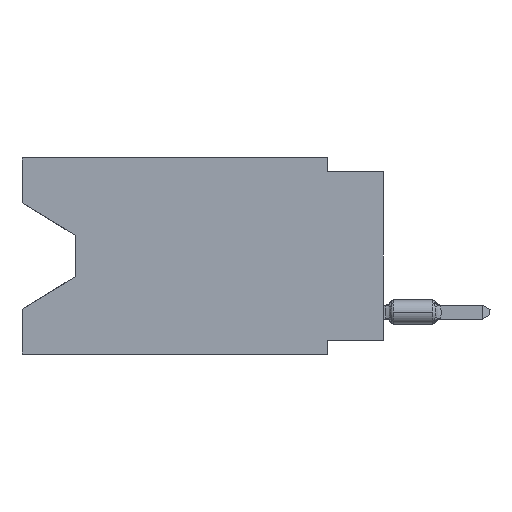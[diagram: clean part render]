
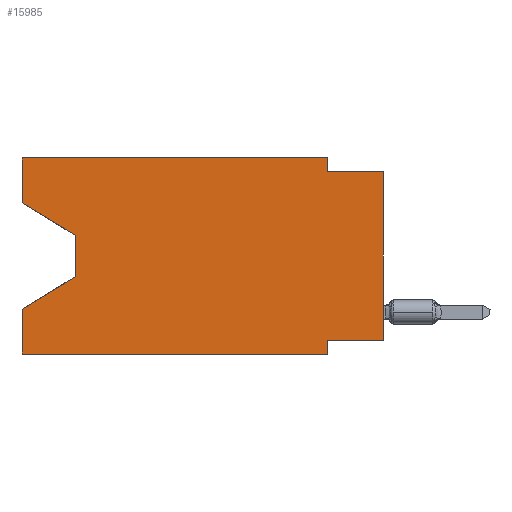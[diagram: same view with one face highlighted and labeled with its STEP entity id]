
A CAD part, left-side view. The second image highlights one B-rep face of the part: STEP entity #15985.
In plain terms, the highlighted planar face has unit normal (-1, 0, 0).
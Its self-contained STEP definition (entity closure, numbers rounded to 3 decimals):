
#483 = VECTOR ( 'NONE', #1953, 1000. ) ;
#767 = VECTOR ( 'NONE', #28940, 1000. ) ;
#1034 = EDGE_CURVE ( 'NONE', #12911, #21335, #12960, .T. ) ;
#1428 = DIRECTION ( 'NONE',  ( 0., 0., -1. ) ) ;
#1506 = DIRECTION ( 'NONE',  ( 0., 1., 0. ) ) ;
#1793 = LINE ( 'NONE', #39458, #31166 ) ;
#1870 = ORIENTED_EDGE ( 'NONE', *, *, #17593, .F. ) ;
#1953 = DIRECTION ( 'NONE',  ( 0., 0., -1. ) ) ;
#2510 = VECTOR ( 'NONE', #7330, 1000. ) ;
#3344 = ORIENTED_EDGE ( 'NONE', *, *, #20951, .T. ) ;
#3581 = CARTESIAN_POINT ( 'NONE',  ( 0., 16.383, 0. ) ) ;
#4400 = VERTEX_POINT ( 'NONE', #16969 ) ;
#4441 = CARTESIAN_POINT ( 'NONE',  ( 0., 0., -8.255 ) ) ;
#5203 = PLANE ( 'NONE',  #10796 ) ;
#5470 = VECTOR ( 'NONE', #10614, 1000. ) ;
#5656 = EDGE_CURVE ( 'NONE', #24074, #6248, #36336, .T. ) ;
#6248 = VERTEX_POINT ( 'NONE', #31164 ) ;
#6799 = CARTESIAN_POINT ( 'NONE',  ( 0., 16.383, -2.038 ) ) ;
#7330 = DIRECTION ( 'NONE',  ( 0., 0., 1. ) ) ;
#7397 = ORIENTED_EDGE ( 'NONE', *, *, #16352, .F. ) ;
#7588 = VERTEX_POINT ( 'NONE', #18638 ) ;
#8215 = LINE ( 'NONE', #37264, #33104 ) ;
#8838 = VERTEX_POINT ( 'NONE', #21826 ) ;
#9325 = ORIENTED_EDGE ( 'NONE', *, *, #1034, .F. ) ;
#10462 = CARTESIAN_POINT ( 'NONE',  ( 0., 0., 0. ) ) ;
#10614 = DIRECTION ( 'NONE',  ( 0., -1., 0. ) ) ;
#10796 = AXIS2_PLACEMENT_3D ( 'NONE', #24029, #27588, #30504 ) ;
#11314 = EDGE_CURVE ( 'NONE', #30246, #21335, #15968, .T. ) ;
#12759 = CARTESIAN_POINT ( 'NONE',  ( 0., 2.54, -8.89 ) ) ;
#12911 = VERTEX_POINT ( 'NONE', #27607 ) ;
#12960 = LINE ( 'NONE', #12759, #27134 ) ;
#13256 = DIRECTION ( 'NONE',  ( 0., 0.855, -0.519 ) ) ;
#13585 = CARTESIAN_POINT ( 'NONE',  ( 0., 13.97, -3.505 ) ) ;
#13607 = LINE ( 'NONE', #10462, #2510 ) ;
#15098 = ORIENTED_EDGE ( 'NONE', *, *, #11314, .T. ) ;
#15968 = LINE ( 'NONE', #19528, #767 ) ;
#15985 = ADVANCED_FACE ( 'NONE', ( #39509 ), #5203, .F. ) ;
#16352 = EDGE_CURVE ( 'NONE', #4400, #34290, #35697, .T. ) ;
#16667 = ORIENTED_EDGE ( 'NONE', *, *, #29815, .F. ) ;
#16969 = CARTESIAN_POINT ( 'NONE',  ( 0., 2.54, -0.635 ) ) ;
#17593 = EDGE_CURVE ( 'NONE', #30246, #25131, #32216, .T. ) ;
#18638 = CARTESIAN_POINT ( 'NONE',  ( 0., 0., -8.255 ) ) ;
#19528 = CARTESIAN_POINT ( 'NONE',  ( 0., 16.383, -8.89 ) ) ;
#19959 = CARTESIAN_POINT ( 'NONE',  ( 0., 13.97, -5.385 ) ) ;
#20731 = VERTEX_POINT ( 'NONE', #33976 ) ;
#20875 = VECTOR ( 'NONE', #32410, 1000. ) ;
#20951 = EDGE_CURVE ( 'NONE', #6248, #25131, #23508, .T. ) ;
#21134 = CARTESIAN_POINT ( 'NONE',  ( 0., 0., -0.635 ) ) ;
#21335 = VERTEX_POINT ( 'NONE', #29323 ) ;
#21826 = CARTESIAN_POINT ( 'NONE',  ( 0., 16.383, 0. ) ) ;
#21961 = ORIENTED_EDGE ( 'NONE', *, *, #30308, .F. ) ;
#22131 = EDGE_CURVE ( 'NONE', #20731, #24074, #33102, .T. ) ;
#23314 = CARTESIAN_POINT ( 'NONE',  ( 0., 16.383, -8.89 ) ) ;
#23508 = LINE ( 'NONE', #19959, #36705 ) ;
#23607 = VECTOR ( 'NONE', #1428, 1000. ) ;
#23843 = ORIENTED_EDGE ( 'NONE', *, *, #32200, .T. ) ;
#24029 = CARTESIAN_POINT ( 'NONE',  ( 0., 16.383, 0. ) ) ;
#24074 = VERTEX_POINT ( 'NONE', #13585 ) ;
#25131 = VERTEX_POINT ( 'NONE', #33535 ) ;
#25135 = ORIENTED_EDGE ( 'NONE', *, *, #22131, .T. ) ;
#25252 = ORIENTED_EDGE ( 'NONE', *, *, #5656, .T. ) ;
#27110 = DIRECTION ( 'NONE',  ( 0., -1., 0. ) ) ;
#27134 = VECTOR ( 'NONE', #31162, 1000. ) ;
#27588 = DIRECTION ( 'NONE',  ( 1., 0., 0. ) ) ;
#27607 = CARTESIAN_POINT ( 'NONE',  ( 0., 2.54, -8.255 ) ) ;
#28354 = CARTESIAN_POINT ( 'NONE',  ( 0., 2.54, 0. ) ) ;
#28828 = EDGE_CURVE ( 'NONE', #20731, #8838, #8215, .T. ) ;
#28940 = DIRECTION ( 'NONE',  ( 0., -1., 0. ) ) ;
#29106 = CARTESIAN_POINT ( 'NONE',  ( 0., 13.97, -3.505 ) ) ;
#29323 = CARTESIAN_POINT ( 'NONE',  ( 0., 2.54, -8.89 ) ) ;
#29815 = EDGE_CURVE ( 'NONE', #8838, #29944, #1793, .T. ) ;
#29944 = VERTEX_POINT ( 'NONE', #28354 ) ;
#30059 = ORIENTED_EDGE ( 'NONE', *, *, #28828, .F. ) ;
#30246 = VERTEX_POINT ( 'NONE', #23314 ) ;
#30308 = EDGE_CURVE ( 'NONE', #29944, #4400, #40007, .T. ) ;
#30504 = DIRECTION ( 'NONE',  ( 0., 0., -1. ) ) ;
#30610 = CARTESIAN_POINT ( 'NONE',  ( 0., 2.54, 0. ) ) ;
#31162 = DIRECTION ( 'NONE',  ( 0., 0., -1. ) ) ;
#31164 = CARTESIAN_POINT ( 'NONE',  ( 0., 13.97, -5.385 ) ) ;
#31166 = VECTOR ( 'NONE', #27110, 1000. ) ;
#31465 = EDGE_LOOP ( 'NONE', ( #25135, #25252, #3344, #1870, #15098, #9325, #38560, #23843, #7397, #21961, #16667, #30059 ) ) ;
#31837 = EDGE_CURVE ( 'NONE', #7588, #12911, #39358, .T. ) ;
#32200 = EDGE_CURVE ( 'NONE', #7588, #34290, #13607, .T. ) ;
#32216 = LINE ( 'NONE', #3581, #20875 ) ;
#32410 = DIRECTION ( 'NONE',  ( 0., 0., 1. ) ) ;
#33102 = LINE ( 'NONE', #6799, #37920 ) ;
#33104 = VECTOR ( 'NONE', #40203, 1000. ) ;
#33279 = VECTOR ( 'NONE', #1506, 1000. ) ;
#33535 = CARTESIAN_POINT ( 'NONE',  ( 0., 16.383, -6.852 ) ) ;
#33976 = CARTESIAN_POINT ( 'NONE',  ( 0., 16.383, -2.038 ) ) ;
#34290 = VERTEX_POINT ( 'NONE', #21134 ) ;
#35279 = CARTESIAN_POINT ( 'NONE',  ( 0., 0., -0.635 ) ) ;
#35697 = LINE ( 'NONE', #35279, #5470 ) ;
#36250 = DIRECTION ( 'NONE',  ( 0., -0.855, -0.519 ) ) ;
#36336 = LINE ( 'NONE', #29106, #23607 ) ;
#36705 = VECTOR ( 'NONE', #13256, 1000. ) ;
#37264 = CARTESIAN_POINT ( 'NONE',  ( 0., 16.383, 0. ) ) ;
#37920 = VECTOR ( 'NONE', #36250, 1000. ) ;
#38560 = ORIENTED_EDGE ( 'NONE', *, *, #31837, .F. ) ;
#39358 = LINE ( 'NONE', #4441, #33279 ) ;
#39458 = CARTESIAN_POINT ( 'NONE',  ( 0., 16.383, 0. ) ) ;
#39509 = FACE_OUTER_BOUND ( 'NONE', #31465, .T. ) ;
#40007 = LINE ( 'NONE', #30610, #483 ) ;
#40203 = DIRECTION ( 'NONE',  ( 0., 0., 1. ) ) ;
